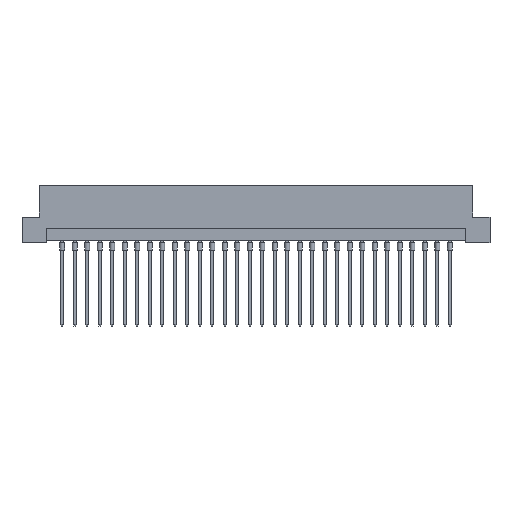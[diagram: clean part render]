
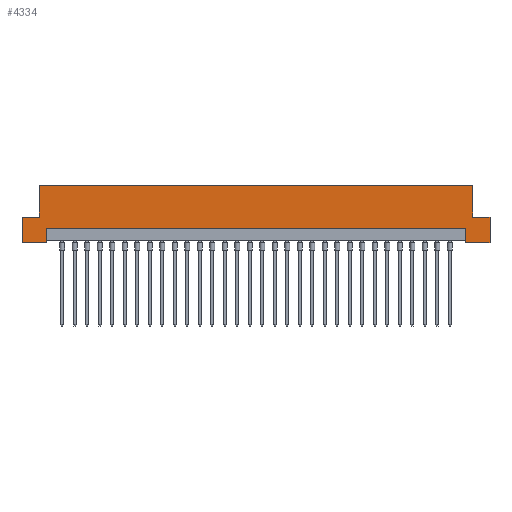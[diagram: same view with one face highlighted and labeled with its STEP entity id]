
A CAD part, front view. The second image highlights one B-rep face of the part: STEP entity #4334.
In plain terms, the highlighted planar face has unit normal (0, -1, 0).
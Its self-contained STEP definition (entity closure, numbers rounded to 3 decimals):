
#66 = CARTESIAN_POINT ( 'NONE',  ( 44., 0., 11.6 ) ) ;
#316 = DIRECTION ( 'NONE',  ( 0., 0., -1. ) ) ;
#432 = CARTESIAN_POINT ( 'NONE',  ( 47.5, 0., 0. ) ) ;
#830 = LINE ( 'NONE', #13867, #1353 ) ;
#853 = VECTOR ( 'NONE', #6608, 1000. ) ;
#1018 = CARTESIAN_POINT ( 'NONE',  ( 47.5, 0., 0. ) ) ;
#1327 = ORIENTED_EDGE ( 'NONE', *, *, #15114, .T. ) ;
#1353 = VECTOR ( 'NONE', #8198, 1000. ) ;
#1462 = CARTESIAN_POINT ( 'NONE',  ( -47.5, 0., 0. ) ) ;
#1577 = VECTOR ( 'NONE', #2165, 1000. ) ;
#1890 = FACE_OUTER_BOUND ( 'NONE', #16468, .T. ) ;
#2130 = VERTEX_POINT ( 'NONE', #12975 ) ;
#2165 = DIRECTION ( 'NONE',  ( 0., 0., 1. ) ) ;
#2351 = LINE ( 'NONE', #12192, #853 ) ;
#2363 = CARTESIAN_POINT ( 'NONE',  ( 44., 0., 5.2 ) ) ;
#2515 = VERTEX_POINT ( 'NONE', #2560 ) ;
#2560 = CARTESIAN_POINT ( 'NONE',  ( -47.5, 0., 5.2 ) ) ;
#2765 = CARTESIAN_POINT ( 'NONE',  ( 42.6, 0., 0.5 ) ) ;
#3015 = DIRECTION ( 'NONE',  ( -1., 0., 0. ) ) ;
#3040 = EDGE_CURVE ( 'NONE', #14002, #17995, #2351, .T. ) ;
#3344 = LINE ( 'NONE', #432, #4361 ) ;
#3401 = VECTOR ( 'NONE', #15863, 1000. ) ;
#3576 = LINE ( 'NONE', #17994, #1577 ) ;
#3794 = ORIENTED_EDGE ( 'NONE', *, *, #8684, .F. ) ;
#4129 = EDGE_CURVE ( 'NONE', #5936, #11102, #8515, .T. ) ;
#4334 = ADVANCED_FACE ( 'NONE', ( #1890 ), #10490, .F. ) ;
#4361 = VECTOR ( 'NONE', #16133, 1000. ) ;
#4367 = EDGE_CURVE ( 'NONE', #12300, #8887, #7554, .T. ) ;
#4393 = DIRECTION ( 'NONE',  ( 0., 0., -1. ) ) ;
#4397 = ORIENTED_EDGE ( 'NONE', *, *, #6759, .F. ) ;
#4762 = CARTESIAN_POINT ( 'NONE',  ( -44., 0., 11.6 ) ) ;
#5031 = VERTEX_POINT ( 'NONE', #10745 ) ;
#5100 = VERTEX_POINT ( 'NONE', #11219 ) ;
#5283 = LINE ( 'NONE', #2363, #16598 ) ;
#5689 = VECTOR ( 'NONE', #4393, 1000. ) ;
#5729 = CARTESIAN_POINT ( 'NONE',  ( -47.5, 0., 5.2 ) ) ;
#5763 = LINE ( 'NONE', #15989, #6530 ) ;
#5936 = VERTEX_POINT ( 'NONE', #6059 ) ;
#6054 = VECTOR ( 'NONE', #7748, 1000. ) ;
#6059 = CARTESIAN_POINT ( 'NONE',  ( -42.6, 0., 0. ) ) ;
#6530 = VECTOR ( 'NONE', #3015, 1000. ) ;
#6608 = DIRECTION ( 'NONE',  ( 1., 0., 0. ) ) ;
#6759 = EDGE_CURVE ( 'NONE', #2515, #2130, #8397, .T. ) ;
#6926 = VECTOR ( 'NONE', #11535, 1000. ) ;
#7121 = VECTOR ( 'NONE', #15014, 1000. ) ;
#7421 = CARTESIAN_POINT ( 'NONE',  ( -42.6, 0., 0.5 ) ) ;
#7531 = ORIENTED_EDGE ( 'NONE', *, *, #4129, .F. ) ;
#7554 = LINE ( 'NONE', #17997, #6054 ) ;
#7748 = DIRECTION ( 'NONE',  ( -1., 0., 0. ) ) ;
#8198 = DIRECTION ( 'NONE',  ( 0., 0., 1. ) ) ;
#8397 = LINE ( 'NONE', #5729, #3401 ) ;
#8515 = LINE ( 'NONE', #12959, #6926 ) ;
#8684 = EDGE_CURVE ( 'NONE', #2130, #14002, #830, .T. ) ;
#8852 = VERTEX_POINT ( 'NONE', #12914 ) ;
#8887 = VERTEX_POINT ( 'NONE', #13183 ) ;
#8899 = EDGE_CURVE ( 'NONE', #17125, #12300, #3344, .T. ) ;
#8918 = LINE ( 'NONE', #2765, #12812 ) ;
#9243 = LINE ( 'NONE', #18067, #7121 ) ;
#9263 = CARTESIAN_POINT ( 'NONE',  ( -47.5, 0., 11.6 ) ) ;
#9543 = ORIENTED_EDGE ( 'NONE', *, *, #10005, .F. ) ;
#10005 = EDGE_CURVE ( 'NONE', #5031, #5100, #5763, .T. ) ;
#10081 = ORIENTED_EDGE ( 'NONE', *, *, #14333, .T. ) ;
#10481 = ORIENTED_EDGE ( 'NONE', *, *, #4367, .F. ) ;
#10490 = PLANE ( 'NONE',  #18416 ) ;
#10745 = CARTESIAN_POINT ( 'NONE',  ( 42.6, 0., 2.9 ) ) ;
#11102 = VERTEX_POINT ( 'NONE', #1462 ) ;
#11219 = CARTESIAN_POINT ( 'NONE',  ( -42.6, 0., 2.9 ) ) ;
#11535 = DIRECTION ( 'NONE',  ( -1., 0., 0. ) ) ;
#11704 = EDGE_CURVE ( 'NONE', #11102, #2515, #3576, .T. ) ;
#12140 = ORIENTED_EDGE ( 'NONE', *, *, #8899, .F. ) ;
#12192 = CARTESIAN_POINT ( 'NONE',  ( -47.5, 0., 11.6 ) ) ;
#12300 = VERTEX_POINT ( 'NONE', #1018 ) ;
#12812 = VECTOR ( 'NONE', #316, 1000. ) ;
#12914 = CARTESIAN_POINT ( 'NONE',  ( 44., 0., 5.2 ) ) ;
#12959 = CARTESIAN_POINT ( 'NONE',  ( -47.5, 0., 0. ) ) ;
#12975 = CARTESIAN_POINT ( 'NONE',  ( -44., 0., 5.2 ) ) ;
#13183 = CARTESIAN_POINT ( 'NONE',  ( 42.6, 0., 0. ) ) ;
#13456 = EDGE_CURVE ( 'NONE', #8852, #17125, #9243, .T. ) ;
#13867 = CARTESIAN_POINT ( 'NONE',  ( -44., 0., 5.2 ) ) ;
#14002 = VERTEX_POINT ( 'NONE', #4762 ) ;
#14333 = EDGE_CURVE ( 'NONE', #5031, #8887, #8918, .T. ) ;
#14409 = ORIENTED_EDGE ( 'NONE', *, *, #3040, .F. ) ;
#14855 = CARTESIAN_POINT ( 'NONE',  ( 47.5, 0., 5.2 ) ) ;
#15014 = DIRECTION ( 'NONE',  ( 1., 0., 0. ) ) ;
#15114 = EDGE_CURVE ( 'NONE', #8852, #17995, #5283, .T. ) ;
#15863 = DIRECTION ( 'NONE',  ( 1., 0., 0. ) ) ;
#15989 = CARTESIAN_POINT ( 'NONE',  ( 42.6, 0., 2.9 ) ) ;
#16049 = ORIENTED_EDGE ( 'NONE', *, *, #11704, .F. ) ;
#16133 = DIRECTION ( 'NONE',  ( 0., 0., -1. ) ) ;
#16278 = DIRECTION ( 'NONE',  ( 0., 0., 1. ) ) ;
#16336 = LINE ( 'NONE', #7421, #5689 ) ;
#16468 = EDGE_LOOP ( 'NONE', ( #9543, #10081, #10481, #12140, #17745, #1327, #14409, #3794, #4397, #16049, #7531, #18313 ) ) ;
#16476 = DIRECTION ( 'NONE',  ( 0., 1., 0. ) ) ;
#16598 = VECTOR ( 'NONE', #16667, 1000. ) ;
#16667 = DIRECTION ( 'NONE',  ( 0., 0., 1. ) ) ;
#17125 = VERTEX_POINT ( 'NONE', #14855 ) ;
#17745 = ORIENTED_EDGE ( 'NONE', *, *, #13456, .F. ) ;
#17994 = CARTESIAN_POINT ( 'NONE',  ( -47.5, 0., 0. ) ) ;
#17995 = VERTEX_POINT ( 'NONE', #66 ) ;
#17997 = CARTESIAN_POINT ( 'NONE',  ( -47.5, 0., 0. ) ) ;
#18067 = CARTESIAN_POINT ( 'NONE',  ( 47.5, 0., 5.2 ) ) ;
#18237 = EDGE_CURVE ( 'NONE', #5100, #5936, #16336, .T. ) ;
#18313 = ORIENTED_EDGE ( 'NONE', *, *, #18237, .F. ) ;
#18416 = AXIS2_PLACEMENT_3D ( 'NONE', #9263, #16476, #16278 ) ;
